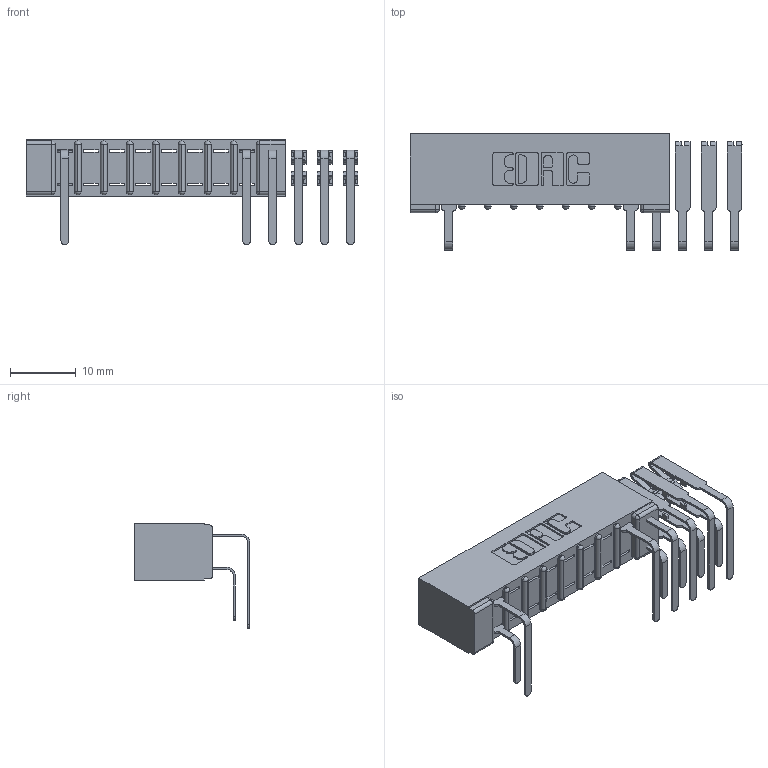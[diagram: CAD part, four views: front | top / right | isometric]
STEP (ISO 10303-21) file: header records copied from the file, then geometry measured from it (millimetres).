
FILE_DESCRIPTION (( 'STEP AP203' ), '1' );
FILE_NAME ('357-024-559-201.STEP', '2018-08-09T01:20:55', ( '' ), ( '' ), 'SwSTEP 2.0', 'SolidWorks 2016', '' );
FILE_SCHEMA (( 'CONFIG_CONTROL_DESIGN' ));
Length unit declared in the file: inch
Products named in the file (4): 307 Part_No Mounting Lugs; 307-290-001_558 559 - 1 (Single); 307-290-001_559 - 2 (Single); 357-024-559-201
Assembly tree (12 placements, depth 2):
  357-024-559-201
    307 Part_No Mounting Lugs
    307-290-001_558 559 - 1 (Single)  x5
    307-290-001_559 - 2 (Single)  x6
Bounding box: 50.63 x 17.69 x 16.08 mm (x, y, z)
Volume: 2808.9 mm3; surface area: 4603.9 mm2
Topology: 12 solids, 12 shells, 719 faces, 2021 edges, 1306 vertices
Faces by surface type: plane 459, cylinder 242, sphere 18
Entity records: 12315 total; most frequent: CARTESIAN_POINT 2045, ORIENTED_EDGE 2026, DIRECTION 2011, EDGE_CURVE 1013, LINE 763, VECTOR 763, VERTEX_POINT 658, AXIS2_PLACEMENT_3D 624
